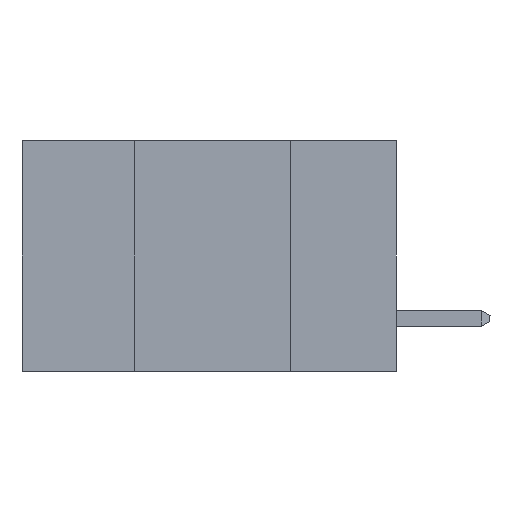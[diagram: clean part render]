
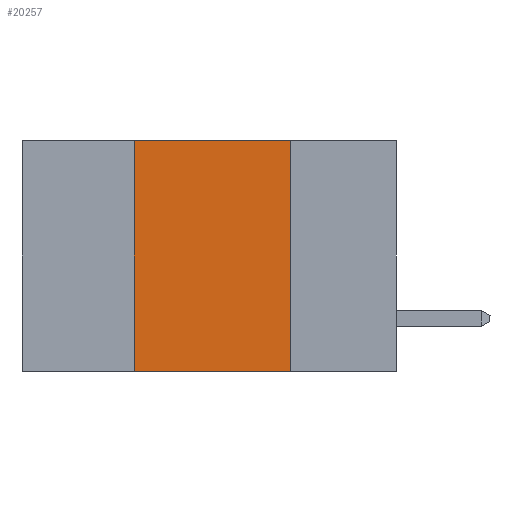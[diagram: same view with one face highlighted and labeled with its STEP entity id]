
A CAD part, left-side view. The second image highlights one B-rep face of the part: STEP entity #20257.
In plain terms, the highlighted planar face has unit normal (-1, 0, 0).
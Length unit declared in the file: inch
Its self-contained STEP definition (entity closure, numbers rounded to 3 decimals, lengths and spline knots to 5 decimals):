
#1920 = LINE ( 'NONE', #5866, #16718 ) ;
#2216 = DIRECTION ( 'NONE',  ( 0., 0., -1. ) ) ;
#3033 = CARTESIAN_POINT ( 'NONE',  ( 0., 0.17, -0.37 ) ) ;
#3391 = EDGE_CURVE ( 'NONE', #22214, #20768, #12312, .T. ) ;
#3946 = DIRECTION ( 'NONE',  ( 0., -1., 0. ) ) ;
#4743 = EDGE_CURVE ( 'NONE', #20768, #11105, #14077, .T. ) ;
#5821 = ORIENTED_EDGE ( 'NONE', *, *, #3391, .F. ) ;
#5866 = CARTESIAN_POINT ( 'NONE',  ( 0., 0.6, -0.37 ) ) ;
#5902 = CARTESIAN_POINT ( 'NONE',  ( 0., 0.6, 0. ) ) ;
#7808 = PLANE ( 'NONE',  #21284 ) ;
#10380 = CARTESIAN_POINT ( 'NONE',  ( 0., 0.42, -0.37 ) ) ;
#10390 = DIRECTION ( 'NONE',  ( 0., 0., -1. ) ) ;
#11105 = VERTEX_POINT ( 'NONE', #13783 ) ;
#11739 = DIRECTION ( 'NONE',  ( 1., 0., 0. ) ) ;
#12312 = LINE ( 'NONE', #13953, #17045 ) ;
#13756 = CARTESIAN_POINT ( 'NONE',  ( 0., 0.42, -0.37 ) ) ;
#13783 = CARTESIAN_POINT ( 'NONE',  ( 0., 0.17, -0.37 ) ) ;
#13822 = EDGE_CURVE ( 'NONE', #23865, #22214, #21948, .T. ) ;
#13953 = CARTESIAN_POINT ( 'NONE',  ( 0., 0.6, 0. ) ) ;
#14077 = LINE ( 'NONE', #3033, #20082 ) ;
#16097 = DIRECTION ( 'NONE',  ( 0., 0., 1. ) ) ;
#16718 = VECTOR ( 'NONE', #3946, 39.37008 ) ;
#17045 = VECTOR ( 'NONE', #19785, 39.37008 ) ;
#17651 = EDGE_CURVE ( 'NONE', #23865, #11105, #1920, .T. ) ;
#19785 = DIRECTION ( 'NONE',  ( 0., -1., 0. ) ) ;
#19821 = CARTESIAN_POINT ( 'NONE',  ( 0., 0.17, 0. ) ) ;
#20082 = VECTOR ( 'NONE', #10390, 39.37008 ) ;
#20257 = ADVANCED_FACE ( 'NONE', ( #21766 ), #7808, .F. ) ;
#20587 = ORIENTED_EDGE ( 'NONE', *, *, #4743, .F. ) ;
#20768 = VERTEX_POINT ( 'NONE', #19821 ) ;
#21232 = ORIENTED_EDGE ( 'NONE', *, *, #13822, .F. ) ;
#21284 = AXIS2_PLACEMENT_3D ( 'NONE', #5902, #11739, #2216 ) ;
#21766 = FACE_OUTER_BOUND ( 'NONE', #24895, .T. ) ;
#21928 = VECTOR ( 'NONE', #16097, 39.37008 ) ;
#21948 = LINE ( 'NONE', #10380, #21928 ) ;
#22214 = VERTEX_POINT ( 'NONE', #23778 ) ;
#23778 = CARTESIAN_POINT ( 'NONE',  ( 0., 0.42, 0. ) ) ;
#23865 = VERTEX_POINT ( 'NONE', #13756 ) ;
#24706 = ORIENTED_EDGE ( 'NONE', *, *, #17651, .T. ) ;
#24895 = EDGE_LOOP ( 'NONE', ( #20587, #5821, #21232, #24706 ) ) ;
